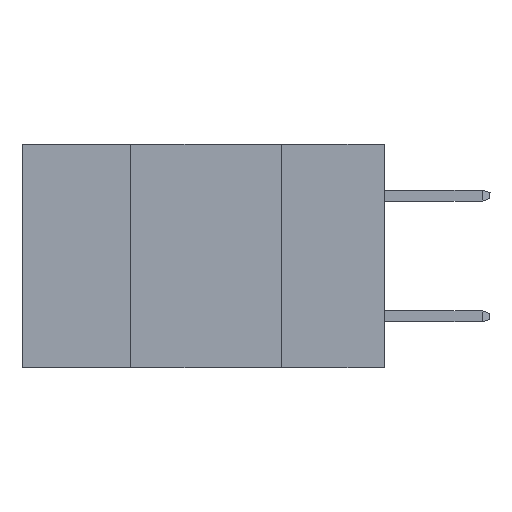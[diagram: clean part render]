
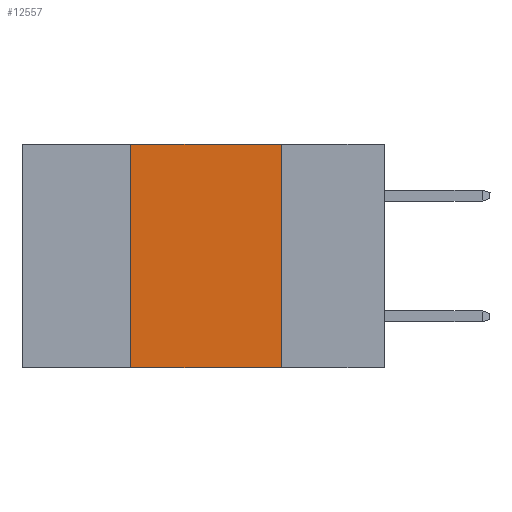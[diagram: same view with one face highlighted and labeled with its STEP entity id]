
A CAD part, left-side view. The second image highlights one B-rep face of the part: STEP entity #12557.
In plain terms, the highlighted planar face has unit normal (-1, 0, 0).
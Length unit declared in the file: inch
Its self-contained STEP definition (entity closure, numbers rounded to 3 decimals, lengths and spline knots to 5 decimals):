
#100 = VERTEX_POINT ( 'NONE', #878 ) ;
#503 = VECTOR ( 'NONE', #7793, 39.37008 ) ;
#733 = VECTOR ( 'NONE', #16421, 39.37008 ) ;
#878 = CARTESIAN_POINT ( 'NONE',  ( 0., 0.42, 0. ) ) ;
#1736 = VERTEX_POINT ( 'NONE', #19380 ) ;
#1858 = CARTESIAN_POINT ( 'NONE',  ( 0., 0.6, 0. ) ) ;
#2196 = DIRECTION ( 'NONE',  ( 1., 0., 0. ) ) ;
#2283 = VECTOR ( 'NONE', #7864, 39.37008 ) ;
#2588 = LINE ( 'NONE', #8442, #733 ) ;
#4518 = CARTESIAN_POINT ( 'NONE',  ( 0., 0.17, 0. ) ) ;
#5471 = FACE_OUTER_BOUND ( 'NONE', #24792, .T. ) ;
#6561 = LINE ( 'NONE', #19734, #9993 ) ;
#6581 = ORIENTED_EDGE ( 'NONE', *, *, #16832, .T. ) ;
#6765 = ORIENTED_EDGE ( 'NONE', *, *, #17828, .F. ) ;
#7212 = VERTEX_POINT ( 'NONE', #4518 ) ;
#7793 = DIRECTION ( 'NONE',  ( 0., 0., -1. ) ) ;
#7864 = DIRECTION ( 'NONE',  ( 0., 0., 1. ) ) ;
#7931 = DIRECTION ( 'NONE',  ( 0., -1., 0. ) ) ;
#8063 = CARTESIAN_POINT ( 'NONE',  ( 0., 0.17, 0. ) ) ;
#8442 = CARTESIAN_POINT ( 'NONE',  ( 0., 0.6, -0.37 ) ) ;
#9993 = VECTOR ( 'NONE', #7931, 39.37008 ) ;
#9998 = DIRECTION ( 'NONE',  ( 0., 0., -1. ) ) ;
#10504 = CARTESIAN_POINT ( 'NONE',  ( 0., 0.17, -0.37 ) ) ;
#12557 = ADVANCED_FACE ( 'NONE', ( #5471 ), #19784, .F. ) ;
#12888 = EDGE_CURVE ( 'NONE', #7212, #19462, #19397, .T. ) ;
#14701 = ORIENTED_EDGE ( 'NONE', *, *, #20606, .F. ) ;
#16421 = DIRECTION ( 'NONE',  ( 0., -1., 0. ) ) ;
#16556 = LINE ( 'NONE', #17772, #2283 ) ;
#16832 = EDGE_CURVE ( 'NONE', #1736, #19462, #2588, .T. ) ;
#17760 = ORIENTED_EDGE ( 'NONE', *, *, #12888, .F. ) ;
#17772 = CARTESIAN_POINT ( 'NONE',  ( 0., 0.42, 0. ) ) ;
#17828 = EDGE_CURVE ( 'NONE', #100, #7212, #6561, .T. ) ;
#19380 = CARTESIAN_POINT ( 'NONE',  ( 0., 0.42, -0.37 ) ) ;
#19397 = LINE ( 'NONE', #8063, #503 ) ;
#19462 = VERTEX_POINT ( 'NONE', #10504 ) ;
#19734 = CARTESIAN_POINT ( 'NONE',  ( 0., 0.6, 0. ) ) ;
#19784 = PLANE ( 'NONE',  #22559 ) ;
#20606 = EDGE_CURVE ( 'NONE', #1736, #100, #16556, .T. ) ;
#22559 = AXIS2_PLACEMENT_3D ( 'NONE', #1858, #2196, #9998 ) ;
#24792 = EDGE_LOOP ( 'NONE', ( #17760, #6765, #14701, #6581 ) ) ;
